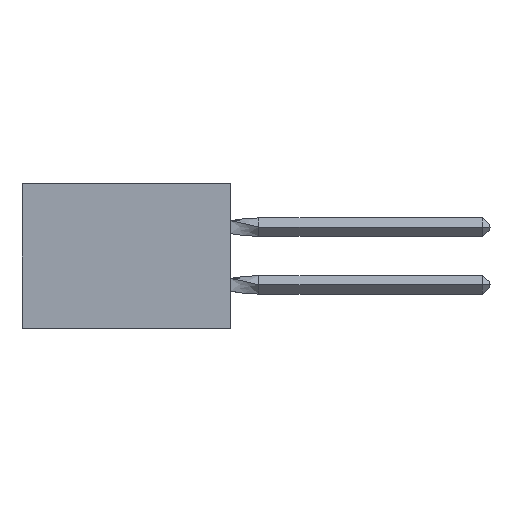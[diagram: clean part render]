
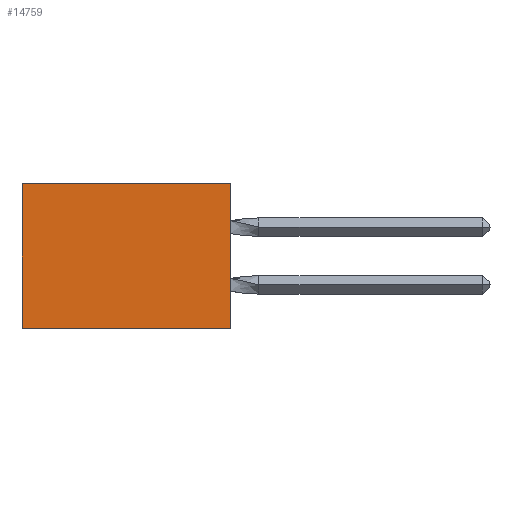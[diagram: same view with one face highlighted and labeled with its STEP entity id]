
A CAD part, left-side view. The second image highlights one B-rep face of the part: STEP entity #14759.
In plain terms, the highlighted planar face has unit normal (-1, 0, 0).
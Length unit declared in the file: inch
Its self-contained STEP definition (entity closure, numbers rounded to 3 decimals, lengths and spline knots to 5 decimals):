
#52 = ORIENTED_EDGE ( 'NONE', *, *, #18756, .F. ) ;
#290 = CARTESIAN_POINT ( 'NONE',  ( 0.305, 0., 0. ) ) ;
#1457 = CARTESIAN_POINT ( 'NONE',  ( 0.305, 0., -0.5 ) ) ;
#1683 = AXIS2_PLACEMENT_3D ( 'NONE', #1457, #5039, #22371 ) ;
#4022 = CARTESIAN_POINT ( 'NONE',  ( 0.305, 0., 0. ) ) ;
#4464 = ORIENTED_EDGE ( 'NONE', *, *, #15324, .F. ) ;
#4882 = VERTEX_POINT ( 'NONE', #19291 ) ;
#5039 = DIRECTION ( 'NONE',  ( 1., 0., 0. ) ) ;
#5375 = CARTESIAN_POINT ( 'NONE',  ( 0.305, 0.72, -0.5 ) ) ;
#6225 = VERTEX_POINT ( 'NONE', #7182 ) ;
#6691 = VERTEX_POINT ( 'NONE', #4022 ) ;
#6960 = VECTOR ( 'NONE', #7758, 39.37008 ) ;
#7182 = CARTESIAN_POINT ( 'NONE',  ( 0.305, 0., -0.5 ) ) ;
#7371 = ORIENTED_EDGE ( 'NONE', *, *, #15087, .T. ) ;
#7758 = DIRECTION ( 'NONE',  ( 0., 1., 0. ) ) ;
#8772 = VECTOR ( 'NONE', #21576, 39.37008 ) ;
#9044 = VECTOR ( 'NONE', #9122, 39.37008 ) ;
#9122 = DIRECTION ( 'NONE',  ( 0., 0., -1. ) ) ;
#10399 = LINE ( 'NONE', #5375, #9044 ) ;
#10635 = LINE ( 'NONE', #290, #8772 ) ;
#10794 = ORIENTED_EDGE ( 'NONE', *, *, #20647, .T. ) ;
#11296 = VERTEX_POINT ( 'NONE', #17543 ) ;
#11581 = LINE ( 'NONE', #16472, #6960 ) ;
#13032 = VECTOR ( 'NONE', #13259, 39.37008 ) ;
#13259 = DIRECTION ( 'NONE',  ( 0., 0., -1. ) ) ;
#14387 = LINE ( 'NONE', #21725, #13032 ) ;
#14759 = ADVANCED_FACE ( 'NONE', ( #21732 ), #18690, .F. ) ;
#15087 = EDGE_CURVE ( 'NONE', #6691, #4882, #10635, .T. ) ;
#15324 = EDGE_CURVE ( 'NONE', #6691, #6225, #14387, .T. ) ;
#16472 = CARTESIAN_POINT ( 'NONE',  ( 0.305, 0., -0.5 ) ) ;
#17543 = CARTESIAN_POINT ( 'NONE',  ( 0.305, 0.72, -0.5 ) ) ;
#18690 = PLANE ( 'NONE',  #1683 ) ;
#18756 = EDGE_CURVE ( 'NONE', #6225, #11296, #11581, .T. ) ;
#19291 = CARTESIAN_POINT ( 'NONE',  ( 0.305, 0.72, 0. ) ) ;
#20647 = EDGE_CURVE ( 'NONE', #4882, #11296, #10399, .T. ) ;
#21043 = EDGE_LOOP ( 'NONE', ( #10794, #52, #4464, #7371 ) ) ;
#21576 = DIRECTION ( 'NONE',  ( 0., 1., 0. ) ) ;
#21725 = CARTESIAN_POINT ( 'NONE',  ( 0.305, 0., -0.5 ) ) ;
#21732 = FACE_OUTER_BOUND ( 'NONE', #21043, .T. ) ;
#22371 = DIRECTION ( 'NONE',  ( 0., 0., -1. ) ) ;
